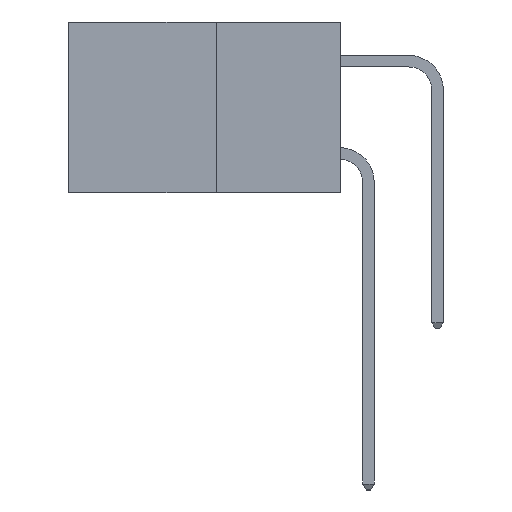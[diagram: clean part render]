
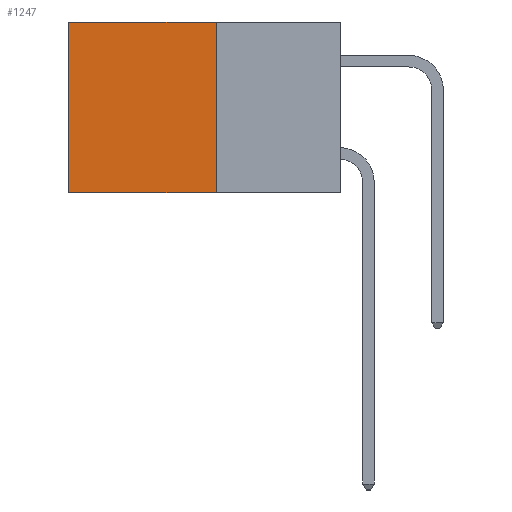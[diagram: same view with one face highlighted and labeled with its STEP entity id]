
A CAD part, left-side view. The second image highlights one B-rep face of the part: STEP entity #1247.
In plain terms, the highlighted planar face has unit normal (-1, 0, 0).
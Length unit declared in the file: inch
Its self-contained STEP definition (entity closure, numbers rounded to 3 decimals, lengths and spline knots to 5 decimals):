
#276 = CARTESIAN_POINT ( 'NONE',  ( 0.277, 0.27, 0. ) ) ;
#603 = DIRECTION ( 'NONE',  ( 0., 1., 0. ) ) ;
#918 = LINE ( 'NONE', #2857, #5442 ) ;
#1159 = VERTEX_POINT ( 'NONE', #8614 ) ;
#1247 = ADVANCED_FACE ( 'NONE', ( #5619 ), #6736, .F. ) ;
#1261 = ORIENTED_EDGE ( 'NONE', *, *, #1793, .F. ) ;
#1663 = VECTOR ( 'NONE', #2303, 39.37008 ) ;
#1793 = EDGE_CURVE ( 'NONE', #1159, #8779, #918, .T. ) ;
#1914 = EDGE_CURVE ( 'NONE', #5520, #8779, #11256, .T. ) ;
#2118 = LINE ( 'NONE', #11152, #8762 ) ;
#2303 = DIRECTION ( 'NONE',  ( 0., 0., -1. ) ) ;
#2728 = CARTESIAN_POINT ( 'NONE',  ( 0.277, 0.27, -0.37 ) ) ;
#2857 = CARTESIAN_POINT ( 'NONE',  ( 0.277, 0.27, -0.37 ) ) ;
#3128 = DIRECTION ( 'NONE',  ( 0., 0., -1. ) ) ;
#3366 = VECTOR ( 'NONE', #3128, 39.37008 ) ;
#3427 = ORIENTED_EDGE ( 'NONE', *, *, #3536, .T. ) ;
#3536 = EDGE_CURVE ( 'NONE', #4224, #5520, #2118, .T. ) ;
#3653 = DIRECTION ( 'NONE',  ( 1., 0., 0. ) ) ;
#3814 = CARTESIAN_POINT ( 'NONE',  ( 0.277, 0.59, -0.37 ) ) ;
#4208 = CARTESIAN_POINT ( 'NONE',  ( 0.277, 0.59, 0. ) ) ;
#4220 = CARTESIAN_POINT ( 'NONE',  ( 0.277, 0.27, -0.37 ) ) ;
#4224 = VERTEX_POINT ( 'NONE', #276 ) ;
#4919 = CARTESIAN_POINT ( 'NONE',  ( 0.277, 0.59, -0.37 ) ) ;
#5442 = VECTOR ( 'NONE', #603, 39.37008 ) ;
#5520 = VERTEX_POINT ( 'NONE', #4208 ) ;
#5553 = EDGE_CURVE ( 'NONE', #4224, #1159, #6348, .T. ) ;
#5619 = FACE_OUTER_BOUND ( 'NONE', #7339, .T. ) ;
#6348 = LINE ( 'NONE', #2728, #3366 ) ;
#6712 = DIRECTION ( 'NONE',  ( 0., 0., -1. ) ) ;
#6736 = PLANE ( 'NONE',  #8711 ) ;
#7339 = EDGE_LOOP ( 'NONE', ( #10635, #1261, #10363, #3427 ) ) ;
#8614 = CARTESIAN_POINT ( 'NONE',  ( 0.277, 0.27, -0.37 ) ) ;
#8711 = AXIS2_PLACEMENT_3D ( 'NONE', #4220, #3653, #6712 ) ;
#8762 = VECTOR ( 'NONE', #11518, 39.37008 ) ;
#8779 = VERTEX_POINT ( 'NONE', #4919 ) ;
#10363 = ORIENTED_EDGE ( 'NONE', *, *, #5553, .F. ) ;
#10635 = ORIENTED_EDGE ( 'NONE', *, *, #1914, .T. ) ;
#11152 = CARTESIAN_POINT ( 'NONE',  ( 0.277, 0.27, 0. ) ) ;
#11256 = LINE ( 'NONE', #3814, #1663 ) ;
#11518 = DIRECTION ( 'NONE',  ( 0., 1., 0. ) ) ;
